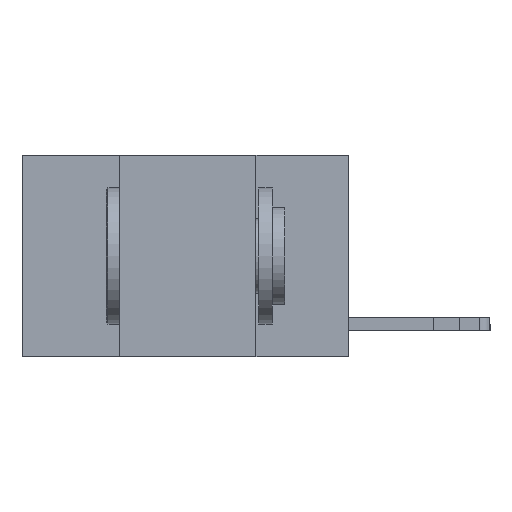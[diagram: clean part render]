
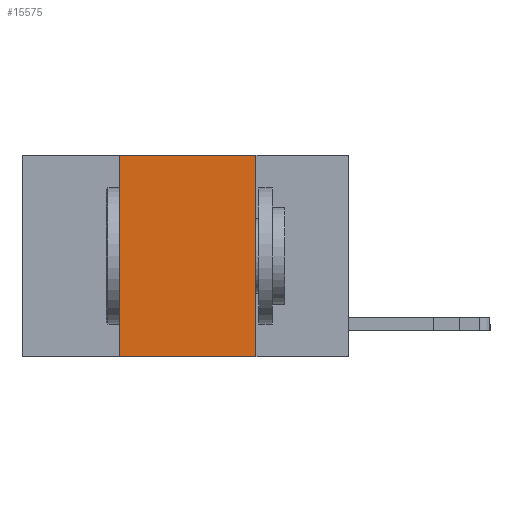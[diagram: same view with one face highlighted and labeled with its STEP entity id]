
A CAD part, left-side view. The second image highlights one B-rep face of the part: STEP entity #15575.
In plain terms, the highlighted planar face has unit normal (-1, 0, 0).
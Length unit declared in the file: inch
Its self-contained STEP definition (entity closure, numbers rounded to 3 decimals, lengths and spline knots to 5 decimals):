
#48 = EDGE_CURVE ( 'NONE', #10671, #14100, #11875, .T. ) ;
#93 = EDGE_CURVE ( 'NONE', #10671, #20386, #19431, .T. ) ;
#1348 = EDGE_CURVE ( 'NONE', #11428, #20386, #10329, .T. ) ;
#1635 = CARTESIAN_POINT ( 'NONE',  ( 0., 0.6, 0. ) ) ;
#2373 = CARTESIAN_POINT ( 'NONE',  ( 0., 0.17, -0.37 ) ) ;
#3296 = DIRECTION ( 'NONE',  ( 0., 0., -1. ) ) ;
#4197 = ORIENTED_EDGE ( 'NONE', *, *, #93, .T. ) ;
#4549 = DIRECTION ( 'NONE',  ( 0., -1., 0. ) ) ;
#4666 = DIRECTION ( 'NONE',  ( 0., 0., -1. ) ) ;
#4910 = CARTESIAN_POINT ( 'NONE',  ( 0., 0.17, 0. ) ) ;
#6627 = DIRECTION ( 'NONE',  ( 0., -1., 0. ) ) ;
#6916 = VECTOR ( 'NONE', #4666, 39.37008 ) ;
#7078 = PLANE ( 'NONE',  #22073 ) ;
#7255 = VECTOR ( 'NONE', #4549, 39.37008 ) ;
#7978 = VECTOR ( 'NONE', #10215, 39.37008 ) ;
#8633 = LINE ( 'NONE', #11838, #13834 ) ;
#8838 = FACE_OUTER_BOUND ( 'NONE', #10463, .T. ) ;
#10215 = DIRECTION ( 'NONE',  ( 0., 0., 1. ) ) ;
#10329 = LINE ( 'NONE', #4910, #6916 ) ;
#10463 = EDGE_LOOP ( 'NONE', ( #12085, #16678, #18125, #4197 ) ) ;
#10671 = VERTEX_POINT ( 'NONE', #17366 ) ;
#11428 = VERTEX_POINT ( 'NONE', #20061 ) ;
#11838 = CARTESIAN_POINT ( 'NONE',  ( 0., 0.6, 0. ) ) ;
#11875 = LINE ( 'NONE', #13657, #7978 ) ;
#12085 = ORIENTED_EDGE ( 'NONE', *, *, #1348, .F. ) ;
#13657 = CARTESIAN_POINT ( 'NONE',  ( 0., 0.42, 0. ) ) ;
#13834 = VECTOR ( 'NONE', #6627, 39.37008 ) ;
#14100 = VERTEX_POINT ( 'NONE', #18789 ) ;
#14299 = DIRECTION ( 'NONE',  ( 1., 0., 0. ) ) ;
#15575 = ADVANCED_FACE ( 'NONE', ( #8838 ), #7078, .F. ) ;
#16678 = ORIENTED_EDGE ( 'NONE', *, *, #19613, .F. ) ;
#17366 = CARTESIAN_POINT ( 'NONE',  ( 0., 0.42, -0.37 ) ) ;
#18125 = ORIENTED_EDGE ( 'NONE', *, *, #48, .F. ) ;
#18789 = CARTESIAN_POINT ( 'NONE',  ( 0., 0.42, 0. ) ) ;
#19431 = LINE ( 'NONE', #20761, #7255 ) ;
#19613 = EDGE_CURVE ( 'NONE', #14100, #11428, #8633, .T. ) ;
#20061 = CARTESIAN_POINT ( 'NONE',  ( 0., 0.17, 0. ) ) ;
#20386 = VERTEX_POINT ( 'NONE', #2373 ) ;
#20761 = CARTESIAN_POINT ( 'NONE',  ( 0., 0.6, -0.37 ) ) ;
#22073 = AXIS2_PLACEMENT_3D ( 'NONE', #1635, #14299, #3296 ) ;
